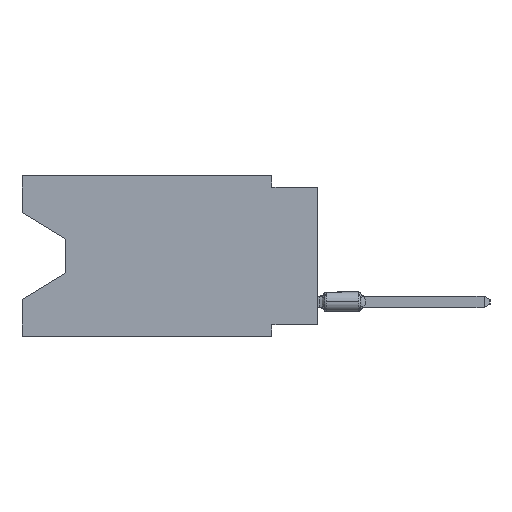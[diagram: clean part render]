
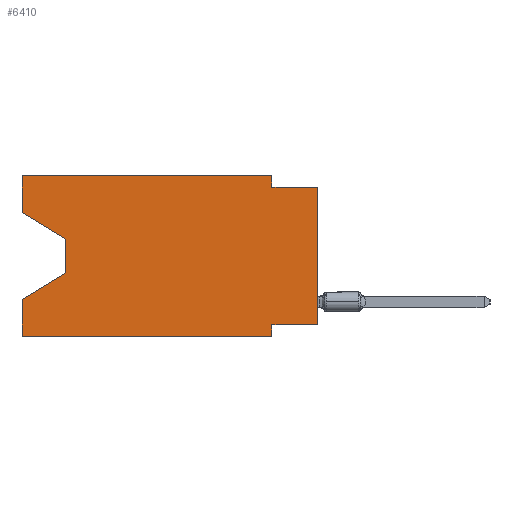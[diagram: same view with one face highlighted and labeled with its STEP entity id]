
A CAD part, left-side view. The second image highlights one B-rep face of the part: STEP entity #6410.
In plain terms, the highlighted planar face has unit normal (-1, 0, 0).
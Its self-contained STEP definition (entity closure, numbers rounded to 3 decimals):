
#106 = DIRECTION ( 'NONE',  ( 0., 0., 1. ) ) ;
#653 = VECTOR ( 'NONE', #2222, 1000. ) ;
#934 = ORIENTED_EDGE ( 'NONE', *, *, #26956, .T. ) ;
#1317 = DIRECTION ( 'NONE',  ( 0., 0., -1. ) ) ;
#2030 = EDGE_CURVE ( 'NONE', #16370, #9048, #17873, .T. ) ;
#2222 = DIRECTION ( 'NONE',  ( 0., 0., 1. ) ) ;
#2273 = ORIENTED_EDGE ( 'NONE', *, *, #16617, .F. ) ;
#3464 = ORIENTED_EDGE ( 'NONE', *, *, #7244, .F. ) ;
#3754 = LINE ( 'NONE', #16180, #27393 ) ;
#3991 = FACE_OUTER_BOUND ( 'NONE', #31924, .T. ) ;
#3999 = VECTOR ( 'NONE', #18041, 1000. ) ;
#4832 = LINE ( 'NONE', #23682, #15577 ) ;
#5050 = CARTESIAN_POINT ( 'NONE',  ( 0., 0., 0. ) ) ;
#5114 = AXIS2_PLACEMENT_3D ( 'NONE', #14371, #24397, #14047 ) ;
#5456 = CARTESIAN_POINT ( 'NONE',  ( 0., 0., -0.635 ) ) ;
#5462 = ORIENTED_EDGE ( 'NONE', *, *, #29826, .F. ) ;
#5646 = VERTEX_POINT ( 'NONE', #13663 ) ;
#5929 = VECTOR ( 'NONE', #106, 1000. ) ;
#5935 = EDGE_CURVE ( 'NONE', #16370, #26219, #21569, .T. ) ;
#5983 = EDGE_CURVE ( 'NONE', #26219, #16476, #7852, .T. ) ;
#6123 = CARTESIAN_POINT ( 'NONE',  ( 0., 16.383, -8.89 ) ) ;
#6209 = VERTEX_POINT ( 'NONE', #17459 ) ;
#6410 = ADVANCED_FACE ( 'NONE', ( #3991 ), #27257, .F. ) ;
#6708 = ORIENTED_EDGE ( 'NONE', *, *, #17201, .F. ) ;
#7112 = LINE ( 'NONE', #5050, #5929 ) ;
#7244 = EDGE_CURVE ( 'NONE', #6209, #5646, #3754, .T. ) ;
#7433 = ORIENTED_EDGE ( 'NONE', *, *, #5983, .T. ) ;
#7852 = LINE ( 'NONE', #24438, #22446 ) ;
#8026 = LINE ( 'NONE', #13291, #14170 ) ;
#8703 = DIRECTION ( 'NONE',  ( 0., 1., 0. ) ) ;
#9048 = VERTEX_POINT ( 'NONE', #10980 ) ;
#9599 = CARTESIAN_POINT ( 'NONE',  ( 0., 2.54, 0. ) ) ;
#9768 = CARTESIAN_POINT ( 'NONE',  ( 0., 13.97, -5.385 ) ) ;
#10096 = LINE ( 'NONE', #9599, #28556 ) ;
#10375 = DIRECTION ( 'NONE',  ( 0., -1., 0. ) ) ;
#10919 = EDGE_CURVE ( 'NONE', #6209, #27932, #7112, .T. ) ;
#10980 = CARTESIAN_POINT ( 'NONE',  ( 0., 16.383, 0. ) ) ;
#11286 = ORIENTED_EDGE ( 'NONE', *, *, #10919, .T. ) ;
#12774 = CARTESIAN_POINT ( 'NONE',  ( 0., 16.383, 0. ) ) ;
#13046 = ORIENTED_EDGE ( 'NONE', *, *, #32116, .F. ) ;
#13291 = CARTESIAN_POINT ( 'NONE',  ( 0., 2.54, -8.89 ) ) ;
#13314 = DIRECTION ( 'NONE',  ( 0., -1., 0. ) ) ;
#13663 = CARTESIAN_POINT ( 'NONE',  ( 0., 2.54, -8.255 ) ) ;
#14047 = DIRECTION ( 'NONE',  ( 0., 0., -1. ) ) ;
#14052 = DIRECTION ( 'NONE',  ( 0., -1., 0. ) ) ;
#14170 = VECTOR ( 'NONE', #23145, 1000. ) ;
#14371 = CARTESIAN_POINT ( 'NONE',  ( 0., 16.383, 0. ) ) ;
#14713 = DIRECTION ( 'NONE',  ( 0., 0.855, -0.519 ) ) ;
#14822 = VERTEX_POINT ( 'NONE', #32388 ) ;
#15174 = CARTESIAN_POINT ( 'NONE',  ( 0., 16.383, -2.038 ) ) ;
#15297 = VECTOR ( 'NONE', #14052, 1000. ) ;
#15577 = VECTOR ( 'NONE', #20307, 1000. ) ;
#15828 = VECTOR ( 'NONE', #14713, 1000. ) ;
#16086 = CARTESIAN_POINT ( 'NONE',  ( 0., 16.383, -8.89 ) ) ;
#16180 = CARTESIAN_POINT ( 'NONE',  ( 0., 0., -8.255 ) ) ;
#16370 = VERTEX_POINT ( 'NONE', #32354 ) ;
#16476 = VERTEX_POINT ( 'NONE', #16918 ) ;
#16617 = EDGE_CURVE ( 'NONE', #18080, #24856, #10096, .T. ) ;
#16918 = CARTESIAN_POINT ( 'NONE',  ( 0., 13.97, -5.385 ) ) ;
#17201 = EDGE_CURVE ( 'NONE', #20413, #18253, #4832, .T. ) ;
#17459 = CARTESIAN_POINT ( 'NONE',  ( 0., 0., -8.255 ) ) ;
#17749 = DIRECTION ( 'NONE',  ( 0., 0., -1. ) ) ;
#17873 = LINE ( 'NONE', #12774, #653 ) ;
#18041 = DIRECTION ( 'NONE',  ( 0., -0.855, -0.519 ) ) ;
#18080 = VERTEX_POINT ( 'NONE', #31747 ) ;
#18253 = VERTEX_POINT ( 'NONE', #20822 ) ;
#18530 = ORIENTED_EDGE ( 'NONE', *, *, #27139, .T. ) ;
#19643 = LINE ( 'NONE', #9768, #15828 ) ;
#20307 = DIRECTION ( 'NONE',  ( 0., 0., 1. ) ) ;
#20413 = VERTEX_POINT ( 'NONE', #6123 ) ;
#20607 = VECTOR ( 'NONE', #10375, 1000. ) ;
#20822 = CARTESIAN_POINT ( 'NONE',  ( 0., 16.383, -6.852 ) ) ;
#21569 = LINE ( 'NONE', #15174, #3999 ) ;
#21863 = LINE ( 'NONE', #16086, #15297 ) ;
#22441 = ORIENTED_EDGE ( 'NONE', *, *, #2030, .F. ) ;
#22446 = VECTOR ( 'NONE', #1317, 1000. ) ;
#23145 = DIRECTION ( 'NONE',  ( 0., 0., -1. ) ) ;
#23285 = CARTESIAN_POINT ( 'NONE',  ( 0., 0., -0.635 ) ) ;
#23682 = CARTESIAN_POINT ( 'NONE',  ( 0., 16.383, 0. ) ) ;
#23885 = LINE ( 'NONE', #29147, #30970 ) ;
#24144 = CARTESIAN_POINT ( 'NONE',  ( 0., 13.97, -3.505 ) ) ;
#24397 = DIRECTION ( 'NONE',  ( 1., 0., 0. ) ) ;
#24438 = CARTESIAN_POINT ( 'NONE',  ( 0., 13.97, -3.505 ) ) ;
#24856 = VERTEX_POINT ( 'NONE', #26685 ) ;
#25616 = ORIENTED_EDGE ( 'NONE', *, *, #28309, .F. ) ;
#26219 = VERTEX_POINT ( 'NONE', #24144 ) ;
#26685 = CARTESIAN_POINT ( 'NONE',  ( 0., 2.54, -0.635 ) ) ;
#26956 = EDGE_CURVE ( 'NONE', #20413, #14822, #21863, .T. ) ;
#27139 = EDGE_CURVE ( 'NONE', #16476, #18253, #19643, .T. ) ;
#27257 = PLANE ( 'NONE',  #5114 ) ;
#27393 = VECTOR ( 'NONE', #8703, 1000. ) ;
#27932 = VERTEX_POINT ( 'NONE', #5456 ) ;
#28309 = EDGE_CURVE ( 'NONE', #9048, #18080, #23885, .T. ) ;
#28537 = LINE ( 'NONE', #23285, #20607 ) ;
#28556 = VECTOR ( 'NONE', #17749, 1000. ) ;
#29147 = CARTESIAN_POINT ( 'NONE',  ( 0., 16.383, 0. ) ) ;
#29826 = EDGE_CURVE ( 'NONE', #24856, #27932, #28537, .T. ) ;
#30970 = VECTOR ( 'NONE', #13314, 1000. ) ;
#31747 = CARTESIAN_POINT ( 'NONE',  ( 0., 2.54, 0. ) ) ;
#31924 = EDGE_LOOP ( 'NONE', ( #33605, #7433, #18530, #6708, #934, #13046, #3464, #11286, #5462, #2273, #25616, #22441 ) ) ;
#32116 = EDGE_CURVE ( 'NONE', #5646, #14822, #8026, .T. ) ;
#32354 = CARTESIAN_POINT ( 'NONE',  ( 0., 16.383, -2.038 ) ) ;
#32388 = CARTESIAN_POINT ( 'NONE',  ( 0., 2.54, -8.89 ) ) ;
#33605 = ORIENTED_EDGE ( 'NONE', *, *, #5935, .T. ) ;
